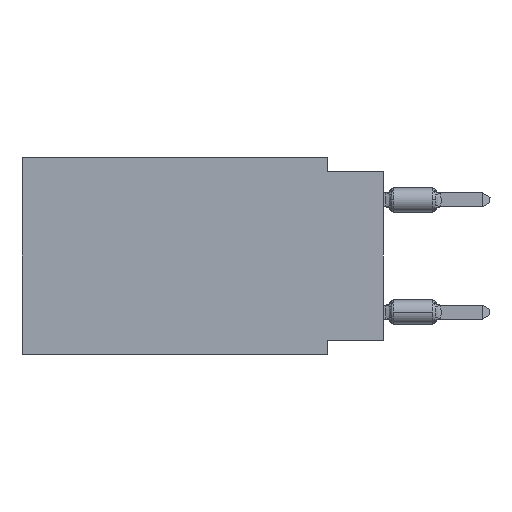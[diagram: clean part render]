
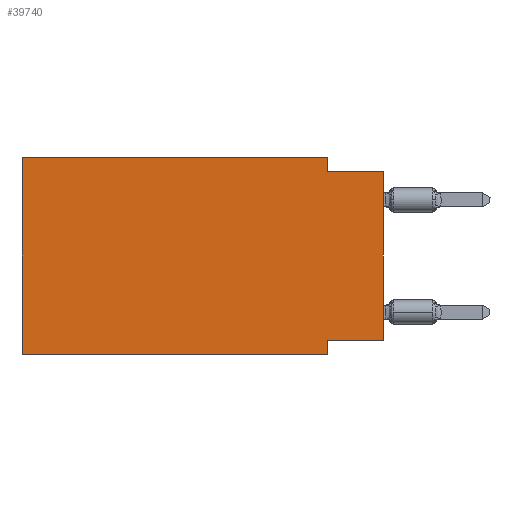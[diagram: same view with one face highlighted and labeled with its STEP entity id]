
A CAD part, left-side view. The second image highlights one B-rep face of the part: STEP entity #39740.
In plain terms, the highlighted planar face has unit normal (-1, 0, 0).
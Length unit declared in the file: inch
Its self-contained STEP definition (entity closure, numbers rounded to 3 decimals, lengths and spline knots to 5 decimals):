
#858 = DIRECTION ( 'NONE',  ( 0., 0., -1. ) ) ;
#1117 = VECTOR ( 'NONE', #37224, 39.37008 ) ;
#1201 = ORIENTED_EDGE ( 'NONE', *, *, #49541, .F. ) ;
#1365 = LINE ( 'NONE', #17733, #1603 ) ;
#1603 = VECTOR ( 'NONE', #9673, 39.37008 ) ;
#2008 = ORIENTED_EDGE ( 'NONE', *, *, #26078, .F. ) ;
#3821 = LINE ( 'NONE', #36587, #23830 ) ;
#3986 = VERTEX_POINT ( 'NONE', #13270 ) ;
#4883 = PLANE ( 'NONE',  #44030 ) ;
#7935 = LINE ( 'NONE', #41508, #1117 ) ;
#8123 = LINE ( 'NONE', #41448, #19952 ) ;
#9673 = DIRECTION ( 'NONE',  ( 0., 0., 1. ) ) ;
#13005 = VERTEX_POINT ( 'NONE', #13362 ) ;
#13270 = CARTESIAN_POINT ( 'NONE',  ( 0., 0.1, -0.35 ) ) ;
#13362 = CARTESIAN_POINT ( 'NONE',  ( 0., 0.645, 0. ) ) ;
#13897 = EDGE_CURVE ( 'NONE', #22605, #33953, #14499, .T. ) ;
#14329 = VECTOR ( 'NONE', #31153, 39.37008 ) ;
#14499 = LINE ( 'NONE', #42984, #14329 ) ;
#15161 = ORIENTED_EDGE ( 'NONE', *, *, #48554, .T. ) ;
#16169 = DIRECTION ( 'NONE',  ( 0., 0., 1. ) ) ;
#17329 = DIRECTION ( 'NONE',  ( 0., -1., 0. ) ) ;
#17733 = CARTESIAN_POINT ( 'NONE',  ( 0., 0., 0. ) ) ;
#18479 = CARTESIAN_POINT ( 'NONE',  ( 0., 0., -0.025 ) ) ;
#19952 = VECTOR ( 'NONE', #36896, 39.37008 ) ;
#20253 = CARTESIAN_POINT ( 'NONE',  ( 0., 0.645, -0.35 ) ) ;
#22019 = ORIENTED_EDGE ( 'NONE', *, *, #51555, .F. ) ;
#22605 = VERTEX_POINT ( 'NONE', #31560 ) ;
#22942 = LINE ( 'NONE', #52220, #30172 ) ;
#23830 = VECTOR ( 'NONE', #16169, 39.37008 ) ;
#23854 = VERTEX_POINT ( 'NONE', #43395 ) ;
#24833 = VERTEX_POINT ( 'NONE', #20253 ) ;
#25560 = DIRECTION ( 'NONE',  ( 1., 0., 0. ) ) ;
#26078 = EDGE_CURVE ( 'NONE', #33953, #52145, #22942, .T. ) ;
#29701 = DIRECTION ( 'NONE',  ( 0., 0., -1. ) ) ;
#30172 = VECTOR ( 'NONE', #39320, 39.37008 ) ;
#31153 = DIRECTION ( 'NONE',  ( 0., 0., -1. ) ) ;
#31560 = CARTESIAN_POINT ( 'NONE',  ( 0., 0.1, 0. ) ) ;
#33953 = VERTEX_POINT ( 'NONE', #41033 ) ;
#36213 = EDGE_CURVE ( 'NONE', #51670, #23854, #8123, .T. ) ;
#36587 = CARTESIAN_POINT ( 'NONE',  ( 0., 0.645, 0. ) ) ;
#36619 = ORIENTED_EDGE ( 'NONE', *, *, #48484, .F. ) ;
#36896 = DIRECTION ( 'NONE',  ( 0., 1., 0. ) ) ;
#37224 = DIRECTION ( 'NONE',  ( 0., -1., 0. ) ) ;
#37750 = CARTESIAN_POINT ( 'NONE',  ( 0., 0.645, -0.35 ) ) ;
#38043 = CARTESIAN_POINT ( 'NONE',  ( 0., 0.1, -0.35 ) ) ;
#38758 = VECTOR ( 'NONE', #17329, 39.37008 ) ;
#38813 = LINE ( 'NONE', #37750, #38758 ) ;
#39320 = DIRECTION ( 'NONE',  ( 0., -1., 0. ) ) ;
#39740 = ADVANCED_FACE ( 'NONE', ( #49754 ), #4883, .F. ) ;
#41033 = CARTESIAN_POINT ( 'NONE',  ( 0., 0.1, -0.025 ) ) ;
#41418 = CARTESIAN_POINT ( 'NONE',  ( 0., 0., -0.325 ) ) ;
#41448 = CARTESIAN_POINT ( 'NONE',  ( 0., 0., -0.325 ) ) ;
#41508 = CARTESIAN_POINT ( 'NONE',  ( 0., 0.645, 0. ) ) ;
#41769 = ORIENTED_EDGE ( 'NONE', *, *, #13897, .F. ) ;
#42572 = ORIENTED_EDGE ( 'NONE', *, *, #50538, .T. ) ;
#42984 = CARTESIAN_POINT ( 'NONE',  ( 0., 0.1, 0. ) ) ;
#43395 = CARTESIAN_POINT ( 'NONE',  ( 0., 0.1, -0.325 ) ) ;
#43586 = ORIENTED_EDGE ( 'NONE', *, *, #36213, .F. ) ;
#44030 = AXIS2_PLACEMENT_3D ( 'NONE', #46233, #25560, #858 ) ;
#46233 = CARTESIAN_POINT ( 'NONE',  ( 0., 0.645, 0. ) ) ;
#47560 = EDGE_LOOP ( 'NONE', ( #42572, #2008, #41769, #36619, #22019, #15161, #1201, #43586 ) ) ;
#48484 = EDGE_CURVE ( 'NONE', #13005, #22605, #7935, .T. ) ;
#48554 = EDGE_CURVE ( 'NONE', #24833, #3986, #38813, .T. ) ;
#49080 = VECTOR ( 'NONE', #29701, 39.37008 ) ;
#49541 = EDGE_CURVE ( 'NONE', #23854, #3986, #49585, .T. ) ;
#49585 = LINE ( 'NONE', #38043, #49080 ) ;
#49754 = FACE_OUTER_BOUND ( 'NONE', #47560, .T. ) ;
#50538 = EDGE_CURVE ( 'NONE', #51670, #52145, #1365, .T. ) ;
#51555 = EDGE_CURVE ( 'NONE', #24833, #13005, #3821, .T. ) ;
#51670 = VERTEX_POINT ( 'NONE', #41418 ) ;
#52145 = VERTEX_POINT ( 'NONE', #18479 ) ;
#52220 = CARTESIAN_POINT ( 'NONE',  ( 0., 0., -0.025 ) ) ;
